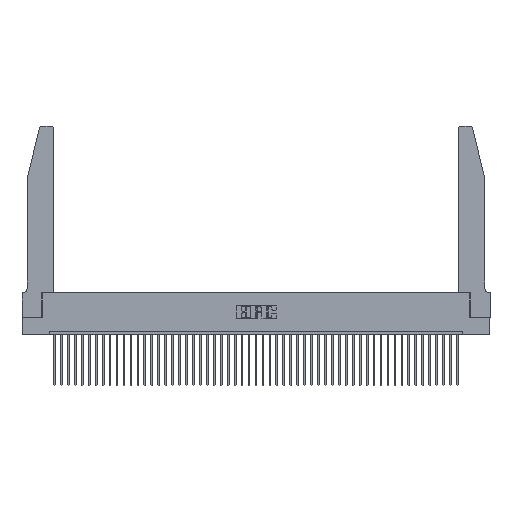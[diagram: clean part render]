
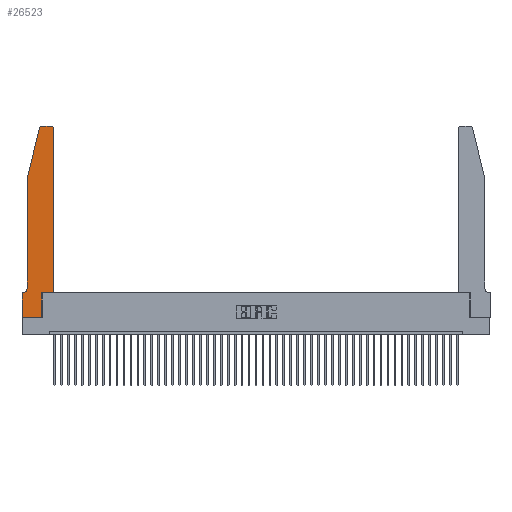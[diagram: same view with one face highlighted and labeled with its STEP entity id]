
A CAD part, top view. The second image highlights one B-rep face of the part: STEP entity #26523.
In plain terms, the highlighted planar face has unit normal (0, 0, 1).
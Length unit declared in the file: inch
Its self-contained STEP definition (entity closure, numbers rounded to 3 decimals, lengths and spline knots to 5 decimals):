
#59 = VECTOR ( 'NONE', #37814, 39.37008 ) ;
#501 = CARTESIAN_POINT ( 'NONE',  ( 0.4505, 0.35, 0.37 ) ) ;
#616 = ORIENTED_EDGE ( 'NONE', *, *, #12034, .T. ) ;
#1080 = EDGE_CURVE ( 'NONE', #43062, #41161, #21250, .T. ) ;
#2292 = CARTESIAN_POINT ( 'NONE',  ( 0., 0., 0.37 ) ) ;
#2681 = CARTESIAN_POINT ( 'NONE',  ( 0.0755, 2., 0.37 ) ) ;
#2925 = LINE ( 'NONE', #39982, #40283 ) ;
#3005 = DIRECTION ( 'NONE',  ( 1., 0., 0. ) ) ;
#3197 = ORIENTED_EDGE ( 'NONE', *, *, #9028, .T. ) ;
#3521 = EDGE_LOOP ( 'NONE', ( #19247, #42596, #35580, #36280, #616, #32329, #32369, #8536, #30508, #3197, #4324, #26571 ) ) ;
#4272 = VECTOR ( 'NONE', #45820, 39.37008 ) ;
#4283 = EDGE_CURVE ( 'NONE', #33463, #31512, #12538, .T. ) ;
#4324 = ORIENTED_EDGE ( 'NONE', *, *, #11539, .T. ) ;
#4419 = DIRECTION ( 'NONE',  ( -0.239, -0.971, 0. ) ) ;
#5632 = AXIS2_PLACEMENT_3D ( 'NONE', #45286, #31051, #31831 ) ;
#5996 = LINE ( 'NONE', #31873, #36005 ) ;
#6855 = CARTESIAN_POINT ( 'NONE',  ( 0., 0., 0.37 ) ) ;
#7235 = FACE_OUTER_BOUND ( 'NONE', #3521, .T. ) ;
#7539 = EDGE_CURVE ( 'NONE', #41832, #43062, #19793, .T. ) ;
#7897 = DIRECTION ( 'NONE',  ( 0., 0., 1. ) ) ;
#8536 = ORIENTED_EDGE ( 'NONE', *, *, #1080, .T. ) ;
#8669 = VERTEX_POINT ( 'NONE', #46346 ) ;
#9028 = EDGE_CURVE ( 'NONE', #8669, #46803, #26392, .T. ) ;
#9121 = VERTEX_POINT ( 'NONE', #45643 ) ;
#9253 = VECTOR ( 'NONE', #45010, 39.37008 ) ;
#9462 = CARTESIAN_POINT ( 'NONE',  ( 0.0755, 2., 0.37 ) ) ;
#11508 = VECTOR ( 'NONE', #12964, 39.37008 ) ;
#11539 = EDGE_CURVE ( 'NONE', #46803, #28356, #36942, .T. ) ;
#12034 = EDGE_CURVE ( 'NONE', #9121, #44457, #35853, .T. ) ;
#12178 = EDGE_CURVE ( 'NONE', #44457, #41832, #2925, .T. ) ;
#12286 = CARTESIAN_POINT ( 'NONE',  ( 0.284, 2.75, 0.37 ) ) ;
#12320 = CARTESIAN_POINT ( 'NONE',  ( 0.4505, 0.35, 0.37 ) ) ;
#12538 = CIRCLE ( 'NONE', #43396, 0.03 ) ;
#12595 = CARTESIAN_POINT ( 'NONE',  ( 0.2865, 0., 0.37 ) ) ;
#12737 = AXIS2_PLACEMENT_3D ( 'NONE', #14032, #24871, #29817 ) ;
#12964 = DIRECTION ( 'NONE',  ( 0., -1., 0. ) ) ;
#13155 = CARTESIAN_POINT ( 'NONE',  ( 0., 0., 0.37 ) ) ;
#14032 = CARTESIAN_POINT ( 'NONE',  ( 0.0055, 0.42, 0.37 ) ) ;
#14347 = LINE ( 'NONE', #9462, #11508 ) ;
#14410 = CARTESIAN_POINT ( 'NONE',  ( 0.4205, 2.75, 0.37 ) ) ;
#15113 = DIRECTION ( 'NONE',  ( 0., 1., 0. ) ) ;
#16596 = VERTEX_POINT ( 'NONE', #2681 ) ;
#16953 = VECTOR ( 'NONE', #15113, 39.37008 ) ;
#17451 = CARTESIAN_POINT ( 'NONE',  ( 0., 0.35, 0.37 ) ) ;
#18364 = EDGE_CURVE ( 'NONE', #16596, #9121, #14347, .T. ) ;
#18870 = CARTESIAN_POINT ( 'NONE',  ( 0.2865, 0.35, 0.37 ) ) ;
#19247 = ORIENTED_EDGE ( 'NONE', *, *, #36613, .T. ) ;
#19548 = DIRECTION ( 'NONE',  ( 0., 0., 1. ) ) ;
#19793 = LINE ( 'NONE', #6855, #59 ) ;
#21250 = LINE ( 'NONE', #2292, #4272 ) ;
#24519 = CARTESIAN_POINT ( 'NONE',  ( 0.284, 2.72, 0.37 ) ) ;
#24871 = DIRECTION ( 'NONE',  ( 0., 0., -1. ) ) ;
#25839 = CARTESIAN_POINT ( 'NONE',  ( 0.4205, 2.72, 0.37 ) ) ;
#26257 = CARTESIAN_POINT ( 'NONE',  ( 0.4505, 0.35, 0.37 ) ) ;
#26392 = LINE ( 'NONE', #26257, #41781 ) ;
#26523 = ADVANCED_FACE ( 'NONE', ( #7235 ), #34379, .T. ) ;
#26571 = ORIENTED_EDGE ( 'NONE', *, *, #40339, .T. ) ;
#28356 = VERTEX_POINT ( 'NONE', #30639 ) ;
#29166 = DIRECTION ( 'NONE',  ( -1., 0., 0. ) ) ;
#29205 = VECTOR ( 'NONE', #4419, 39.37008 ) ;
#29817 = DIRECTION ( 'NONE',  ( -1., 0., 0. ) ) ;
#30508 = ORIENTED_EDGE ( 'NONE', *, *, #44895, .T. ) ;
#30639 = CARTESIAN_POINT ( 'NONE',  ( 0.4505, 2.72, 0.37 ) ) ;
#31051 = DIRECTION ( 'NONE',  ( 0., 0., 1. ) ) ;
#31512 = VERTEX_POINT ( 'NONE', #40665 ) ;
#31652 = LINE ( 'NONE', #18870, #16953 ) ;
#31831 = DIRECTION ( 'NONE',  ( 1., 0., 0. ) ) ;
#31873 = CARTESIAN_POINT ( 'NONE',  ( 0.2605, 2.75, 0.37 ) ) ;
#32329 = ORIENTED_EDGE ( 'NONE', *, *, #12178, .T. ) ;
#32369 = ORIENTED_EDGE ( 'NONE', *, *, #7539, .T. ) ;
#32602 = CARTESIAN_POINT ( 'NONE',  ( 0.0755, 2., 0.37 ) ) ;
#33148 = DIRECTION ( 'NONE',  ( 1., 0., 0. ) ) ;
#33463 = VERTEX_POINT ( 'NONE', #12286 ) ;
#34373 = CIRCLE ( 'NONE', #45237, 0.03 ) ;
#34379 = PLANE ( 'NONE',  #5632 ) ;
#34985 = CARTESIAN_POINT ( 'NONE',  ( 0.0055, 0.35, 0.37 ) ) ;
#35580 = ORIENTED_EDGE ( 'NONE', *, *, #46118, .T. ) ;
#35853 = CIRCLE ( 'NONE', #12737, 0.07 ) ;
#36005 = VECTOR ( 'NONE', #36053, 39.37008 ) ;
#36053 = DIRECTION ( 'NONE',  ( -1., 0., 0. ) ) ;
#36280 = ORIENTED_EDGE ( 'NONE', *, *, #18364, .T. ) ;
#36613 = EDGE_CURVE ( 'NONE', #44780, #33463, #5996, .T. ) ;
#36942 = LINE ( 'NONE', #12320, #9253 ) ;
#37727 = LINE ( 'NONE', #32602, #29205 ) ;
#37814 = DIRECTION ( 'NONE',  ( 0., -1., 0. ) ) ;
#37878 = DIRECTION ( 'NONE',  ( 1., 0., 0. ) ) ;
#39982 = CARTESIAN_POINT ( 'NONE',  ( 0.0755, 0.35, 0.37 ) ) ;
#40283 = VECTOR ( 'NONE', #29166, 39.37008 ) ;
#40339 = EDGE_CURVE ( 'NONE', #28356, #44780, #34373, .T. ) ;
#40665 = CARTESIAN_POINT ( 'NONE',  ( 0.25487, 2.72718, 0.37 ) ) ;
#41161 = VERTEX_POINT ( 'NONE', #12595 ) ;
#41781 = VECTOR ( 'NONE', #37878, 39.37008 ) ;
#41832 = VERTEX_POINT ( 'NONE', #17451 ) ;
#42596 = ORIENTED_EDGE ( 'NONE', *, *, #4283, .T. ) ;
#43062 = VERTEX_POINT ( 'NONE', #13155 ) ;
#43396 = AXIS2_PLACEMENT_3D ( 'NONE', #24519, #19548, #3005 ) ;
#44457 = VERTEX_POINT ( 'NONE', #34985 ) ;
#44780 = VERTEX_POINT ( 'NONE', #14410 ) ;
#44895 = EDGE_CURVE ( 'NONE', #41161, #8669, #31652, .T. ) ;
#45010 = DIRECTION ( 'NONE',  ( 0., 1., 0. ) ) ;
#45237 = AXIS2_PLACEMENT_3D ( 'NONE', #25839, #7897, #33148 ) ;
#45286 = CARTESIAN_POINT ( 'NONE',  ( 0., 0.35, 0.37 ) ) ;
#45643 = CARTESIAN_POINT ( 'NONE',  ( 0.0755, 0.42, 0.37 ) ) ;
#45820 = DIRECTION ( 'NONE',  ( 1., 0., 0. ) ) ;
#46118 = EDGE_CURVE ( 'NONE', #31512, #16596, #37727, .T. ) ;
#46346 = CARTESIAN_POINT ( 'NONE',  ( 0.2865, 0.35, 0.37 ) ) ;
#46803 = VERTEX_POINT ( 'NONE', #501 ) ;
